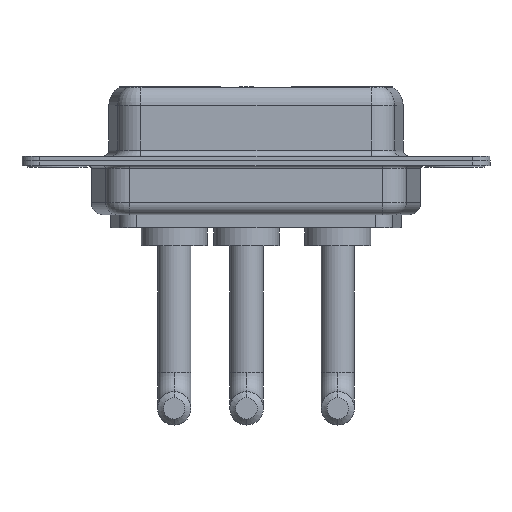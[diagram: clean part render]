
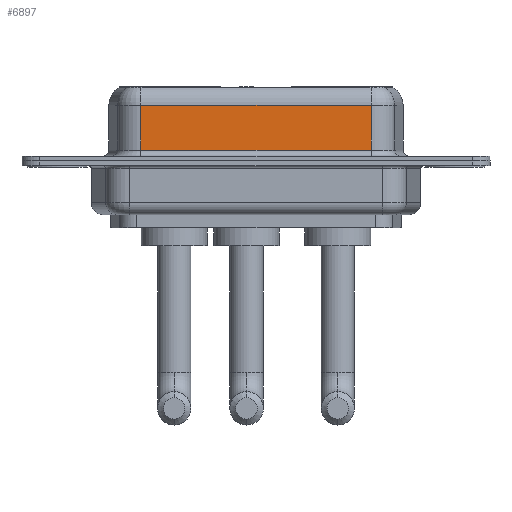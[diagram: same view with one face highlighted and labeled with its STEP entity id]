
A CAD part, front view. The second image highlights one B-rep face of the part: STEP entity #6897.
In plain terms, the highlighted planar face has unit normal (0, -1, 0).
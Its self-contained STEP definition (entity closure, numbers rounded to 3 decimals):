
#299 = AXIS2_PLACEMENT_3D ( 'NONE', #1555, #7023, #638 ) ;
#638 = DIRECTION ( 'NONE',  ( 0., 0., 1. ) ) ;
#689 = VERTEX_POINT ( 'NONE', #7110 ) ;
#731 = LINE ( 'NONE', #2676, #5095 ) ;
#771 = VERTEX_POINT ( 'NONE', #7173 ) ;
#795 = VERTEX_POINT ( 'NONE', #11037 ) ;
#1555 = CARTESIAN_POINT ( 'NONE',  ( 26.287, -3.95, 6.4 ) ) ;
#2291 = LINE ( 'NONE', #6744, #4551 ) ;
#2500 = DIRECTION ( 'NONE',  ( 1., 0., 0. ) ) ;
#2676 = CARTESIAN_POINT ( 'NONE',  ( 26.287, -3.95, 0.9 ) ) ;
#3213 = ORIENTED_EDGE ( 'NONE', *, *, #3878, .T. ) ;
#3347 = ORIENTED_EDGE ( 'NONE', *, *, #11212, .T. ) ;
#3862 = LINE ( 'NONE', #10303, #4033 ) ;
#3878 = EDGE_CURVE ( 'NONE', #795, #771, #731, .T. ) ;
#3913 = ORIENTED_EDGE ( 'NONE', *, *, #8000, .T. ) ;
#4033 = VECTOR ( 'NONE', #11326, 1000. ) ;
#4551 = VECTOR ( 'NONE', #11565, 1000. ) ;
#5095 = VECTOR ( 'NONE', #2500, 1000. ) ;
#5392 = LINE ( 'NONE', #7287, #8988 ) ;
#5543 = EDGE_CURVE ( 'NONE', #11506, #771, #5392, .T. ) ;
#6744 = CARTESIAN_POINT ( 'NONE',  ( 7.013, -3.95, 6.4 ) ) ;
#6897 = ADVANCED_FACE ( 'NONE', ( #7261 ), #9751, .F. ) ;
#6949 = EDGE_LOOP ( 'NONE', ( #7106, #3347, #3913, #3213 ) ) ;
#7023 = DIRECTION ( 'NONE',  ( 0., 1., 0. ) ) ;
#7106 = ORIENTED_EDGE ( 'NONE', *, *, #5543, .F. ) ;
#7110 = CARTESIAN_POINT ( 'NONE',  ( 7.013, -3.95, 4.65 ) ) ;
#7173 = CARTESIAN_POINT ( 'NONE',  ( 26.287, -3.95, 0.9 ) ) ;
#7261 = FACE_OUTER_BOUND ( 'NONE', #6949, .T. ) ;
#7287 = CARTESIAN_POINT ( 'NONE',  ( 26.287, -3.95, 6.4 ) ) ;
#8000 = EDGE_CURVE ( 'NONE', #689, #795, #2291, .T. ) ;
#8140 = DIRECTION ( 'NONE',  ( 0., 0., -1. ) ) ;
#8238 = CARTESIAN_POINT ( 'NONE',  ( 26.287, -3.95, 4.65 ) ) ;
#8988 = VECTOR ( 'NONE', #8140, 1000. ) ;
#9751 = PLANE ( 'NONE',  #299 ) ;
#10303 = CARTESIAN_POINT ( 'NONE',  ( 26.287, -3.95, 4.65 ) ) ;
#11037 = CARTESIAN_POINT ( 'NONE',  ( 7.013, -3.95, 0.9 ) ) ;
#11212 = EDGE_CURVE ( 'NONE', #11506, #689, #3862, .T. ) ;
#11326 = DIRECTION ( 'NONE',  ( -1., 0., 0. ) ) ;
#11506 = VERTEX_POINT ( 'NONE', #8238 ) ;
#11565 = DIRECTION ( 'NONE',  ( 0., 0., -1. ) ) ;
